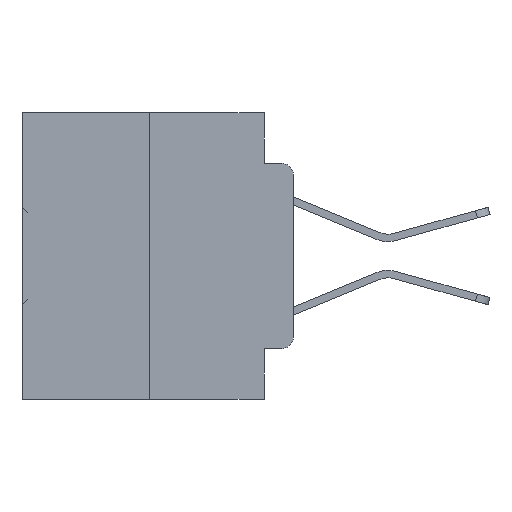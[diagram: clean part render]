
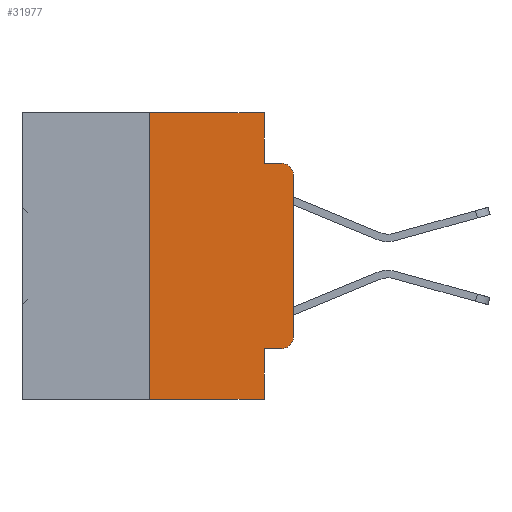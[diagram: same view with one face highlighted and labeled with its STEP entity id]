
A CAD part, left-side view. The second image highlights one B-rep face of the part: STEP entity #31977.
In plain terms, the highlighted planar face has unit normal (-1, 0, 0).
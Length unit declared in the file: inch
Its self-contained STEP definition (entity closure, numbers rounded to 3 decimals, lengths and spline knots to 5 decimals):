
#1189 = CARTESIAN_POINT ( 'NONE',  ( 0., 0.051, -0.4115 ) ) ;
#1231 = DIRECTION ( 'NONE',  ( 0., 0., -1. ) ) ;
#1329 = LINE ( 'NONE', #10599, #6001 ) ;
#1403 = VECTOR ( 'NONE', #23225, 39.37008 ) ;
#1856 = VERTEX_POINT ( 'NONE', #3680 ) ;
#2229 = VERTEX_POINT ( 'NONE', #9212 ) ;
#2587 = CARTESIAN_POINT ( 'NONE',  ( 0., 0.051, 0. ) ) ;
#2900 = VERTEX_POINT ( 'NONE', #23051 ) ;
#3284 = VERTEX_POINT ( 'NONE', #1189 ) ;
#3551 = DIRECTION ( 'NONE',  ( 0., -1., 0. ) ) ;
#3680 = CARTESIAN_POINT ( 'NONE',  ( 0., 0.25, 0. ) ) ;
#3793 = EDGE_CURVE ( 'NONE', #27585, #5158, #21491, .T. ) ;
#4696 = EDGE_CURVE ( 'NONE', #14007, #2900, #13511, .T. ) ;
#5158 = VERTEX_POINT ( 'NONE', #19572 ) ;
#5672 = VECTOR ( 'NONE', #16550, 39.37008 ) ;
#6001 = VECTOR ( 'NONE', #1231, 39.37008 ) ;
#6086 = LINE ( 'NONE', #34579, #33608 ) ;
#6256 = ORIENTED_EDGE ( 'NONE', *, *, #31594, .F. ) ;
#7000 = EDGE_CURVE ( 'NONE', #2229, #27585, #20733, .T. ) ;
#7582 = LINE ( 'NONE', #24200, #25313 ) ;
#8080 = CARTESIAN_POINT ( 'NONE',  ( 0., 0.051, 0. ) ) ;
#8698 = DIRECTION ( 'NONE',  ( 0., 0., -1. ) ) ;
#9212 = CARTESIAN_POINT ( 'NONE',  ( 0., 0.02, -0.4115 ) ) ;
#9575 = ORIENTED_EDGE ( 'NONE', *, *, #37339, .F. ) ;
#9599 = CARTESIAN_POINT ( 'NONE',  ( 0., 0.051, -0.5 ) ) ;
#9938 = FACE_OUTER_BOUND ( 'NONE', #28874, .T. ) ;
#10599 = CARTESIAN_POINT ( 'NONE',  ( 0., 0.051, 0. ) ) ;
#10715 = ORIENTED_EDGE ( 'NONE', *, *, #7000, .T. ) ;
#11147 = LINE ( 'NONE', #29561, #27397 ) ;
#11324 = PLANE ( 'NONE',  #30948 ) ;
#11783 = EDGE_CURVE ( 'NONE', #3284, #28199, #1329, .T. ) ;
#11821 = CARTESIAN_POINT ( 'NONE',  ( 0., 0.051, -0.0885 ) ) ;
#12368 = DIRECTION ( 'NONE',  ( -1., 0., 0. ) ) ;
#12369 = VERTEX_POINT ( 'NONE', #15907 ) ;
#13511 = LINE ( 'NONE', #35397, #1403 ) ;
#14007 = VERTEX_POINT ( 'NONE', #11821 ) ;
#14442 = DIRECTION ( 'NONE',  ( 0., 0., -1. ) ) ;
#15809 = DIRECTION ( 'NONE',  ( 0., -1., 0. ) ) ;
#15907 = CARTESIAN_POINT ( 'NONE',  ( 0., 0.25, -0.5 ) ) ;
#16198 = CARTESIAN_POINT ( 'NONE',  ( 0., 0.473, -0.5 ) ) ;
#16550 = DIRECTION ( 'NONE',  ( 0., 0., 1. ) ) ;
#16556 = VECTOR ( 'NONE', #15809, 39.37008 ) ;
#16898 = DIRECTION ( 'NONE',  ( 0., 0., -1. ) ) ;
#17367 = EDGE_CURVE ( 'NONE', #12369, #28199, #24462, .T. ) ;
#17881 = ORIENTED_EDGE ( 'NONE', *, *, #3793, .T. ) ;
#17993 = EDGE_CURVE ( 'NONE', #3284, #2229, #11147, .T. ) ;
#19572 = CARTESIAN_POINT ( 'NONE',  ( 0., 0., -0.1085 ) ) ;
#19698 = DIRECTION ( 'NONE',  ( 0., 0., 1. ) ) ;
#20407 = DIRECTION ( 'NONE',  ( -1., 0., 0. ) ) ;
#20733 = CIRCLE ( 'NONE', #33033, 0.02 ) ;
#21491 = LINE ( 'NONE', #22768, #5672 ) ;
#22768 = CARTESIAN_POINT ( 'NONE',  ( 0., 0., 0. ) ) ;
#23051 = CARTESIAN_POINT ( 'NONE',  ( 0., 0.02, -0.0885 ) ) ;
#23225 = DIRECTION ( 'NONE',  ( 0., -1., 0. ) ) ;
#23761 = CARTESIAN_POINT ( 'NONE',  ( 0., 0.02, -0.1085 ) ) ;
#23827 = ORIENTED_EDGE ( 'NONE', *, *, #17367, .T. ) ;
#24200 = CARTESIAN_POINT ( 'NONE',  ( 0., 0.473, 0. ) ) ;
#24462 = LINE ( 'NONE', #16198, #16556 ) ;
#24650 = ORIENTED_EDGE ( 'NONE', *, *, #17993, .T. ) ;
#24821 = EDGE_CURVE ( 'NONE', #5158, #2900, #26726, .T. ) ;
#25313 = VECTOR ( 'NONE', #3551, 39.37008 ) ;
#26166 = DIRECTION ( 'NONE',  ( 0., -1., 0. ) ) ;
#26422 = DIRECTION ( 'NONE',  ( 1., 0., 0. ) ) ;
#26726 = CIRCLE ( 'NONE', #35169, 0.02 ) ;
#27397 = VECTOR ( 'NONE', #26166, 39.37008 ) ;
#27585 = VERTEX_POINT ( 'NONE', #33611 ) ;
#28199 = VERTEX_POINT ( 'NONE', #9599 ) ;
#28874 = EDGE_LOOP ( 'NONE', ( #17881, #30913, #36433, #9575, #6256, #34429, #23827, #32749, #24650, #10715 ) ) ;
#29561 = CARTESIAN_POINT ( 'NONE',  ( 0., 0.051, -0.4115 ) ) ;
#29824 = VECTOR ( 'NONE', #37298, 39.37008 ) ;
#30131 = VERTEX_POINT ( 'NONE', #2587 ) ;
#30270 = LINE ( 'NONE', #8080, #29824 ) ;
#30913 = ORIENTED_EDGE ( 'NONE', *, *, #24821, .T. ) ;
#30948 = AXIS2_PLACEMENT_3D ( 'NONE', #32157, #26422, #16898 ) ;
#31594 = EDGE_CURVE ( 'NONE', #1856, #30131, #7582, .T. ) ;
#31977 = ADVANCED_FACE ( 'NONE', ( #9938 ), #11324, .F. ) ;
#32157 = CARTESIAN_POINT ( 'NONE',  ( 0., 0.473, 0. ) ) ;
#32749 = ORIENTED_EDGE ( 'NONE', *, *, #11783, .F. ) ;
#32938 = CARTESIAN_POINT ( 'NONE',  ( 0., 0.02, -0.3915 ) ) ;
#33033 = AXIS2_PLACEMENT_3D ( 'NONE', #32938, #12368, #14442 ) ;
#33608 = VECTOR ( 'NONE', #19698, 39.37008 ) ;
#33611 = CARTESIAN_POINT ( 'NONE',  ( 0., 0., -0.3915 ) ) ;
#34429 = ORIENTED_EDGE ( 'NONE', *, *, #36646, .F. ) ;
#34579 = CARTESIAN_POINT ( 'NONE',  ( 0., 0.25, 0. ) ) ;
#35169 = AXIS2_PLACEMENT_3D ( 'NONE', #23761, #20407, #8698 ) ;
#35397 = CARTESIAN_POINT ( 'NONE',  ( 0., 0.051, -0.0885 ) ) ;
#36433 = ORIENTED_EDGE ( 'NONE', *, *, #4696, .F. ) ;
#36646 = EDGE_CURVE ( 'NONE', #12369, #1856, #6086, .T. ) ;
#37298 = DIRECTION ( 'NONE',  ( 0., 0., -1. ) ) ;
#37339 = EDGE_CURVE ( 'NONE', #30131, #14007, #30270, .T. ) ;
